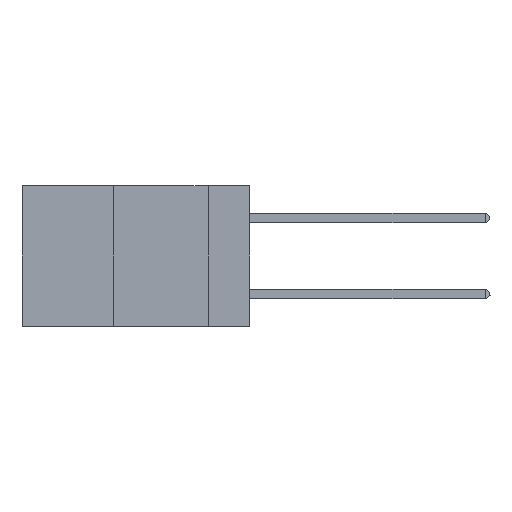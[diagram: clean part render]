
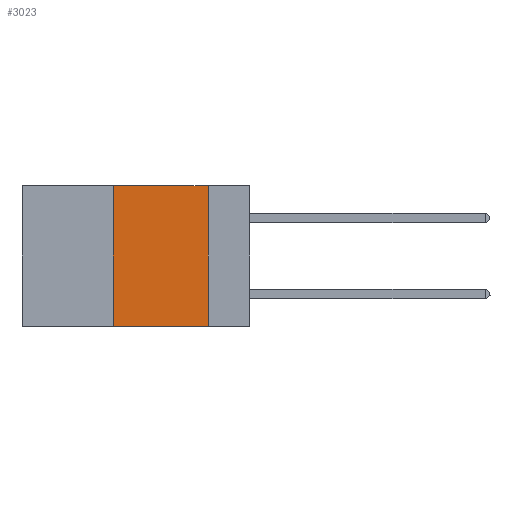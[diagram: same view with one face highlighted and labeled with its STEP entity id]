
A CAD part, left-side view. The second image highlights one B-rep face of the part: STEP entity #3023.
In plain terms, the highlighted planar face has unit normal (-1, 0, 0).
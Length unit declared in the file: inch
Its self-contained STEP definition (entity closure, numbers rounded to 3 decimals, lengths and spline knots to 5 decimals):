
#1092 = VERTEX_POINT ( 'NONE', #26758 ) ;
#2367 = CARTESIAN_POINT ( 'NONE',  ( 0., 0.6, -0.37 ) ) ;
#2739 = FACE_OUTER_BOUND ( 'NONE', #31012, .T. ) ;
#3023 = ADVANCED_FACE ( 'NONE', ( #2739 ), #18876, .F. ) ;
#3184 = CARTESIAN_POINT ( 'NONE',  ( 0., 0.36, 0. ) ) ;
#5686 = CARTESIAN_POINT ( 'NONE',  ( 0., 0.6, 0. ) ) ;
#5913 = DIRECTION ( 'NONE',  ( 0., -1., 0. ) ) ;
#6676 = LINE ( 'NONE', #11048, #14753 ) ;
#7128 = CARTESIAN_POINT ( 'NONE',  ( 0., 0.6, 0. ) ) ;
#8791 = ORIENTED_EDGE ( 'NONE', *, *, #22814, .T. ) ;
#9756 = AXIS2_PLACEMENT_3D ( 'NONE', #5686, #19097, #24531 ) ;
#10615 = VECTOR ( 'NONE', #5913, 39.37008 ) ;
#11048 = CARTESIAN_POINT ( 'NONE',  ( 0., 0.11, 0. ) ) ;
#11390 = ORIENTED_EDGE ( 'NONE', *, *, #14403, .F. ) ;
#12540 = VERTEX_POINT ( 'NONE', #33809 ) ;
#13196 = ORIENTED_EDGE ( 'NONE', *, *, #34133, .F. ) ;
#13548 = DIRECTION ( 'NONE',  ( 0., 0., -1. ) ) ;
#13710 = CARTESIAN_POINT ( 'NONE',  ( 0., 0.36, 0. ) ) ;
#14006 = LINE ( 'NONE', #2367, #10615 ) ;
#14403 = EDGE_CURVE ( 'NONE', #23400, #12540, #25682, .T. ) ;
#14707 = VECTOR ( 'NONE', #14873, 39.37008 ) ;
#14753 = VECTOR ( 'NONE', #13548, 39.37008 ) ;
#14873 = DIRECTION ( 'NONE',  ( 0., -1., 0. ) ) ;
#18876 = PLANE ( 'NONE',  #9756 ) ;
#19097 = DIRECTION ( 'NONE',  ( 1., 0., 0. ) ) ;
#19907 = DIRECTION ( 'NONE',  ( 0., 0., 1. ) ) ;
#20661 = LINE ( 'NONE', #3184, #32945 ) ;
#22814 = EDGE_CURVE ( 'NONE', #24534, #1092, #14006, .T. ) ;
#23400 = VERTEX_POINT ( 'NONE', #13710 ) ;
#24135 = EDGE_CURVE ( 'NONE', #24534, #23400, #20661, .T. ) ;
#24531 = DIRECTION ( 'NONE',  ( 0., 0., -1. ) ) ;
#24534 = VERTEX_POINT ( 'NONE', #32052 ) ;
#25682 = LINE ( 'NONE', #7128, #14707 ) ;
#26758 = CARTESIAN_POINT ( 'NONE',  ( 0., 0.11, -0.37 ) ) ;
#31012 = EDGE_LOOP ( 'NONE', ( #13196, #11390, #33529, #8791 ) ) ;
#32052 = CARTESIAN_POINT ( 'NONE',  ( 0., 0.36, -0.37 ) ) ;
#32945 = VECTOR ( 'NONE', #19907, 39.37008 ) ;
#33529 = ORIENTED_EDGE ( 'NONE', *, *, #24135, .F. ) ;
#33809 = CARTESIAN_POINT ( 'NONE',  ( 0., 0.11, 0. ) ) ;
#34133 = EDGE_CURVE ( 'NONE', #12540, #1092, #6676, .T. ) ;
